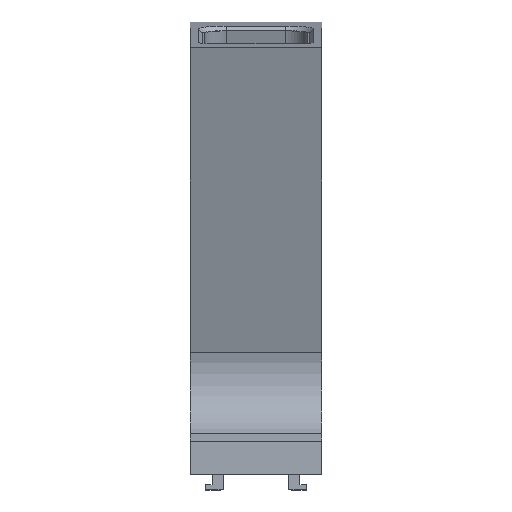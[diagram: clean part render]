
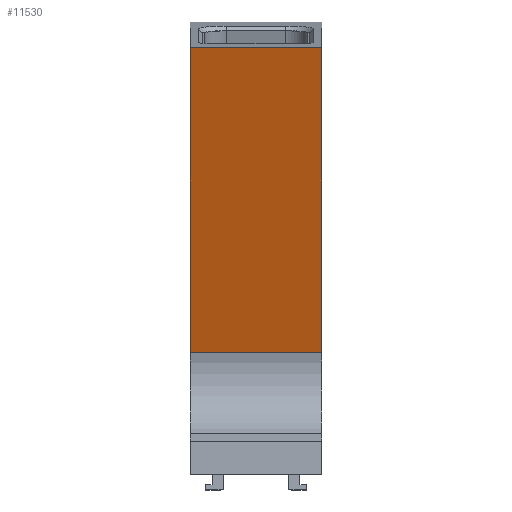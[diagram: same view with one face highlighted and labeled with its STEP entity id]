
A CAD part, left-side view. The second image highlights one B-rep face of the part: STEP entity #11530.
In plain terms, the highlighted planar face has unit normal (-0.951, 0, -0.309).
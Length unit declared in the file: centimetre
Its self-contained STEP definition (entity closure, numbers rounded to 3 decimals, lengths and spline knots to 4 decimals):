
#674=LINE($,#16466,#1463);
#1314=LINE($,#23481,#2103);
#1354=LINE($,#23568,#2143);
#1355=LINE($,#23570,#2144);
#1463=VECTOR($,#13077,3.06);
#2103=VECTOR($,#16089,3.06);
#2143=VECTOR($,#16171,7.4555);
#2144=VECTOR($,#16174,7.4555);
#2342=PLANE($,#12822);
#3090=FACE_OUTER_BOUND($,#3828,.T.);
#3828=EDGE_LOOP($,(#10558,#10559,#10560,#10561));
#4523=VERTEX_POINT($,#16463);
#4524=VERTEX_POINT($,#16465);
#5452=VERTEX_POINT($,#23479);
#5453=VERTEX_POINT($,#23480);
#5607=EDGE_CURVE($,#4523,#4524,#674,.T.);
#7137=EDGE_CURVE($,#5452,#5453,#1314,.T.);
#7183=EDGE_CURVE($,#4524,#5453,#1354,.T.);
#7184=EDGE_CURVE($,#5452,#4523,#1355,.T.);
#10558=ORIENTED_EDGE($,*,*,#5607,.F.);
#10559=ORIENTED_EDGE($,*,*,#7184,.F.);
#10560=ORIENTED_EDGE($,*,*,#7137,.T.);
#10561=ORIENTED_EDGE($,*,*,#7183,.F.);
#11530=ADVANCED_FACE($,(#3090),#2342,.T.);
#12822=AXIS2_PLACEMENT_3D($,#23569,#16172,#16173);
#13077=DIRECTION($,(0.,1.,0.));
#16089=DIRECTION($,(0.,1.,0.));
#16171=DIRECTION($,(-0.309,0.,0.951));
#16172=DIRECTION('center_axis',(-0.951,0.,-0.309));
#16173=DIRECTION('ref_axis',(-0.309,0.,0.951));
#16174=DIRECTION($,(0.309,0.,-0.951));
#16463=CARTESIAN_POINT('',(-6.5495,8.445,-1.1587));
#16465=CARTESIAN_POINT('',(-6.5495,11.505,-1.1587));
#16466=CARTESIAN_POINT($,(-6.5495,9.9632,-1.1587));
#23479=CARTESIAN_POINT('',(-8.8534,8.445,5.9319));
#23480=CARTESIAN_POINT('',(-8.8534,11.505,5.9319));
#23481=CARTESIAN_POINT($,(-8.8534,9.9691,5.9319));
#23568=CARTESIAN_POINT($,(-7.1569,11.505,0.7105));
#23569=CARTESIAN_POINT('Origin',(-8.4963,9.9632,4.8329));
#23570=CARTESIAN_POINT($,(-7.1569,8.445,0.7105));
